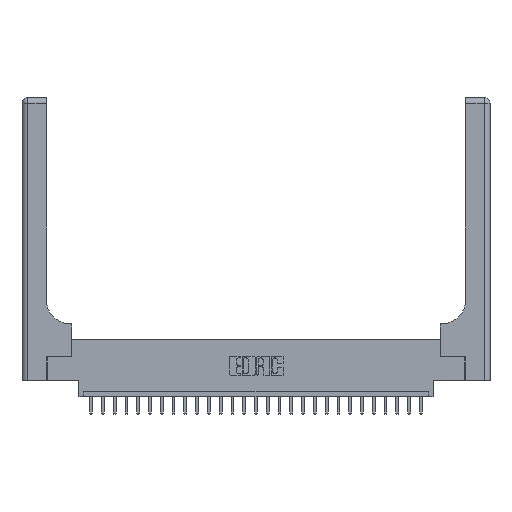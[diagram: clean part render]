
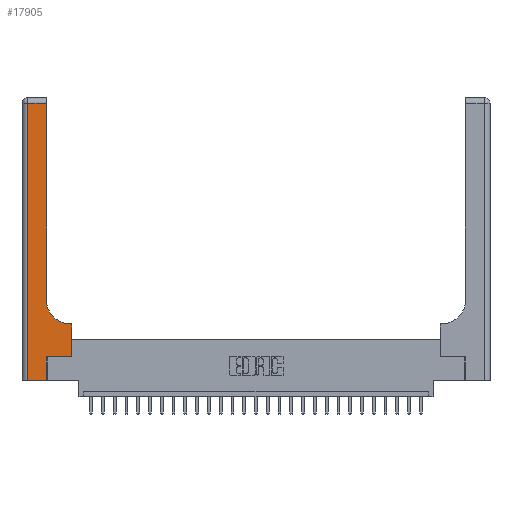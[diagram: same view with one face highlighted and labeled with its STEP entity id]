
A CAD part, top view. The second image highlights one B-rep face of the part: STEP entity #17905.
In plain terms, the highlighted planar face has unit normal (0, 0, 1).
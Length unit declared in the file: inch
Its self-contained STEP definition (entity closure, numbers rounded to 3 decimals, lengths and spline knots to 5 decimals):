
#51 = CARTESIAN_POINT ( 'NONE',  ( 0.528, 0.6, 0.37 ) ) ;
#77 = DIRECTION ( 'NONE',  ( 0., 1., 0. ) ) ;
#650 = AXIS2_PLACEMENT_3D ( 'NONE', #23388, #5643, #21178 ) ;
#866 = VERTEX_POINT ( 'NONE', #8838 ) ;
#904 = VERTEX_POINT ( 'NONE', #12975 ) ;
#936 = EDGE_CURVE ( 'NONE', #24592, #904, #6766, .T. ) ;
#1165 = CARTESIAN_POINT ( 'NONE',  ( 0.265, 0., 0.37 ) ) ;
#1354 = CARTESIAN_POINT ( 'NONE',  ( 0.265, 0.25, 0.37 ) ) ;
#2089 = EDGE_CURVE ( 'NONE', #15078, #11949, #15607, .T. ) ;
#2638 = LINE ( 'NONE', #18679, #16669 ) ;
#3437 = LINE ( 'NONE', #11319, #10366 ) ;
#4007 = VERTEX_POINT ( 'NONE', #13987 ) ;
#4732 = VECTOR ( 'NONE', #14825, 39.37008 ) ;
#4764 = EDGE_CURVE ( 'NONE', #20495, #24894, #19091, .T. ) ;
#4960 = CARTESIAN_POINT ( 'NONE',  ( 0., 3., 0.37 ) ) ;
#4975 = DIRECTION ( 'NONE',  ( 0., 1., 0. ) ) ;
#5337 = ORIENTED_EDGE ( 'NONE', *, *, #14055, .T. ) ;
#5558 = VECTOR ( 'NONE', #11485, 39.37008 ) ;
#5643 = DIRECTION ( 'NONE',  ( 0., 0., -1. ) ) ;
#5672 = LINE ( 'NONE', #5926, #5558 ) ;
#5926 = CARTESIAN_POINT ( 'NONE',  ( 0.06, 3., 0.37 ) ) ;
#5984 = DIRECTION ( 'NONE',  ( 0., 1., 0. ) ) ;
#6766 = LINE ( 'NONE', #12459, #22339 ) ;
#6893 = FACE_OUTER_BOUND ( 'NONE', #8754, .T. ) ;
#7023 = EDGE_CURVE ( 'NONE', #11949, #20495, #3437, .T. ) ;
#7436 = ORIENTED_EDGE ( 'NONE', *, *, #12371, .T. ) ;
#7671 = CIRCLE ( 'NONE', #650, 0.25 ) ;
#8356 = ORIENTED_EDGE ( 'NONE', *, *, #20237, .T. ) ;
#8754 = EDGE_LOOP ( 'NONE', ( #8356, #7436, #15606, #9939, #21585, #10823, #25415, #9388, #5337 ) ) ;
#8838 = CARTESIAN_POINT ( 'NONE',  ( 0.26, 0.85, 0.37 ) ) ;
#9388 = ORIENTED_EDGE ( 'NONE', *, *, #936, .T. ) ;
#9939 = ORIENTED_EDGE ( 'NONE', *, *, #2089, .T. ) ;
#10366 = VECTOR ( 'NONE', #5984, 39.37008 ) ;
#10641 = DIRECTION ( 'NONE',  ( 0., 0., -1. ) ) ;
#10823 = ORIENTED_EDGE ( 'NONE', *, *, #4764, .T. ) ;
#11313 = DIRECTION ( 'NONE',  ( 1., 0., 0. ) ) ;
#11319 = CARTESIAN_POINT ( 'NONE',  ( 0.265, 0., 0.37 ) ) ;
#11485 = DIRECTION ( 'NONE',  ( 0., -1., 0. ) ) ;
#11903 = CARTESIAN_POINT ( 'NONE',  ( 0.265, 0.25, 0.37 ) ) ;
#11949 = VERTEX_POINT ( 'NONE', #1165 ) ;
#12115 = LINE ( 'NONE', #23657, #17467 ) ;
#12371 = EDGE_CURVE ( 'NONE', #13514, #4007, #13006, .T. ) ;
#12459 = CARTESIAN_POINT ( 'NONE',  ( 0.26, 0.6, 0.37 ) ) ;
#12975 = CARTESIAN_POINT ( 'NONE',  ( 0.51, 0.6, 0.37 ) ) ;
#13006 = LINE ( 'NONE', #19090, #4732 ) ;
#13092 = PLANE ( 'NONE',  #23980 ) ;
#13514 = VERTEX_POINT ( 'NONE', #16165 ) ;
#13987 = CARTESIAN_POINT ( 'NONE',  ( 0.06, 2.94, 0.37 ) ) ;
#14055 = EDGE_CURVE ( 'NONE', #904, #866, #7671, .T. ) ;
#14825 = DIRECTION ( 'NONE',  ( -1., 0., 0. ) ) ;
#14902 = CARTESIAN_POINT ( 'NONE',  ( 0.06, 0., 0.37 ) ) ;
#15078 = VERTEX_POINT ( 'NONE', #14902 ) ;
#15606 = ORIENTED_EDGE ( 'NONE', *, *, #22184, .T. ) ;
#15607 = LINE ( 'NONE', #17935, #15871 ) ;
#15871 = VECTOR ( 'NONE', #17681, 39.37008 ) ;
#16165 = CARTESIAN_POINT ( 'NONE',  ( 0.26, 2.94, 0.37 ) ) ;
#16669 = VECTOR ( 'NONE', #4975, 39.37008 ) ;
#17467 = VECTOR ( 'NONE', #77, 39.37008 ) ;
#17681 = DIRECTION ( 'NONE',  ( 1., 0., 0. ) ) ;
#17733 = VECTOR ( 'NONE', #11313, 39.37008 ) ;
#17905 = ADVANCED_FACE ( 'NONE', ( #6893 ), #13092, .F. ) ;
#17935 = CARTESIAN_POINT ( 'NONE',  ( 0., 0., 0.37 ) ) ;
#18679 = CARTESIAN_POINT ( 'NONE',  ( 0.528, 0.25, 0.37 ) ) ;
#18808 = DIRECTION ( 'NONE',  ( -1., 0., 0. ) ) ;
#19090 = CARTESIAN_POINT ( 'NONE',  ( 0., 2.94, 0.37 ) ) ;
#19091 = LINE ( 'NONE', #1354, #17733 ) ;
#20237 = EDGE_CURVE ( 'NONE', #866, #13514, #12115, .T. ) ;
#20495 = VERTEX_POINT ( 'NONE', #11903 ) ;
#21178 = DIRECTION ( 'NONE',  ( 1., 0., 0. ) ) ;
#21585 = ORIENTED_EDGE ( 'NONE', *, *, #7023, .T. ) ;
#21590 = EDGE_CURVE ( 'NONE', #24894, #24592, #2638, .T. ) ;
#22184 = EDGE_CURVE ( 'NONE', #4007, #15078, #5672, .T. ) ;
#22339 = VECTOR ( 'NONE', #18808, 39.37008 ) ;
#22459 = CARTESIAN_POINT ( 'NONE',  ( 0.528, 0.25, 0.37 ) ) ;
#22698 = DIRECTION ( 'NONE',  ( -1., 0., 0. ) ) ;
#23388 = CARTESIAN_POINT ( 'NONE',  ( 0.51, 0.85, 0.37 ) ) ;
#23657 = CARTESIAN_POINT ( 'NONE',  ( 0.26, 3., 0.37 ) ) ;
#23980 = AXIS2_PLACEMENT_3D ( 'NONE', #4960, #10641, #22698 ) ;
#24592 = VERTEX_POINT ( 'NONE', #51 ) ;
#24894 = VERTEX_POINT ( 'NONE', #22459 ) ;
#25415 = ORIENTED_EDGE ( 'NONE', *, *, #21590, .T. ) ;
